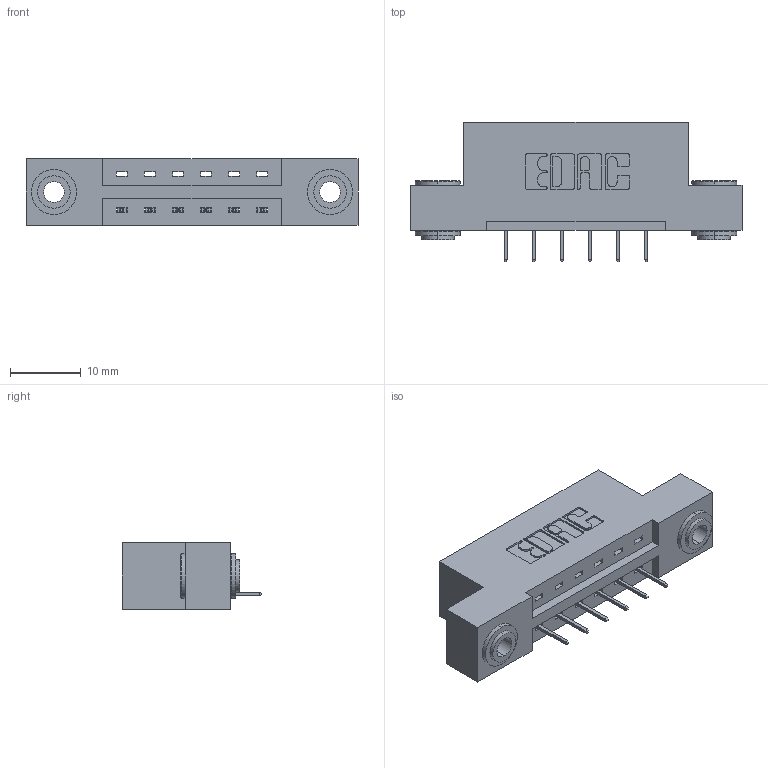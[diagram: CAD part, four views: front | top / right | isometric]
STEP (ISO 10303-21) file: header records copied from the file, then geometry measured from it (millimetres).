
FILE_DESCRIPTION (( 'STEP AP203' ), '1' );
FILE_NAME ('387-006-524-103.STEP', '2019-10-02T00:43:12', ( '' ), ( '' ), 'SwSTEP 2.0', 'SolidWorks 2016', '' );
FILE_SCHEMA (( 'CONFIG_CONTROL_DESIGN' ));
Length unit declared in the file: inch
Products named in the file (4): 387-006-524-103; 345-292-001_345-293-124; 345-250-002_345-250-002-102; 337 Part_Flush Mounting Lugs - 0.156 Dia-TH
Assembly tree (9 placements, depth 2):
  387-006-524-103
    337 Part_Flush Mounting Lugs - 0.156 Dia-TH
    345-292-001_345-293-124  x6
    345-250-002_345-250-002-102  x2
Bounding box: 46.79 x 19.69 x 9.4 mm (x, y, z)
Volume: 4407.9 mm3; surface area: 4504.5 mm2
Topology: 9 solids, 9 shells, 548 faces, 1539 edges, 998 vertices
Faces by surface type: plane 392, cylinder 148, cone 8
Entity records: 9840 total; most frequent: CARTESIAN_POINT 1687, ORIENTED_EDGE 1622, DIRECTION 1529, EDGE_CURVE 811, LINE 663, VECTOR 663, VERTEX_POINT 534, AXIS2_PLACEMENT_3D 433
